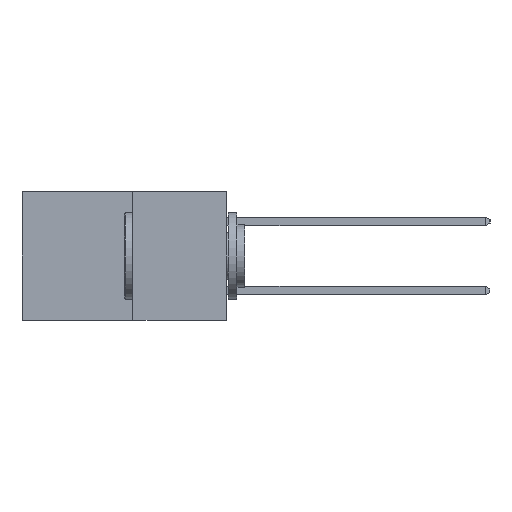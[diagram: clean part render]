
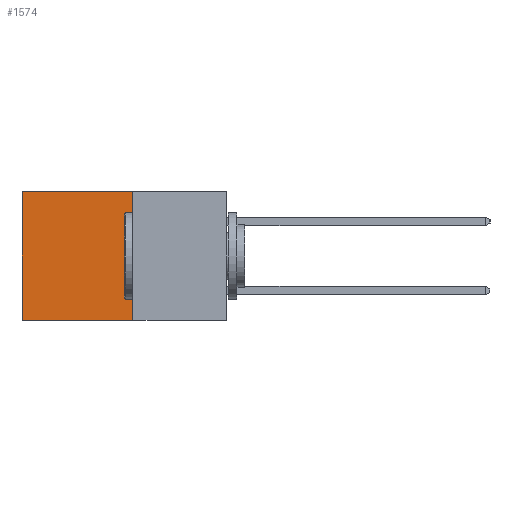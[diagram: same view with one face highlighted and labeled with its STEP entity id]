
A CAD part, left-side view. The second image highlights one B-rep face of the part: STEP entity #1574.
In plain terms, the highlighted planar face has unit normal (-1, 0, 0).
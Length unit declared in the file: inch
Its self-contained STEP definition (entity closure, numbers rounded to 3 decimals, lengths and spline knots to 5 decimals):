
#288 = ORIENTED_EDGE ( 'NONE', *, *, #5386, .F. ) ;
#1240 = VECTOR ( 'NONE', #7402, 39.37008 ) ;
#1245 = EDGE_LOOP ( 'NONE', ( #10589, #288, #12506, #8542 ) ) ;
#1574 = ADVANCED_FACE ( 'NONE', ( #5909 ), #2010, .F. ) ;
#2010 = PLANE ( 'NONE',  #11711 ) ;
#2177 = VECTOR ( 'NONE', #7965, 39.37008 ) ;
#2582 = VERTEX_POINT ( 'NONE', #15142 ) ;
#2954 = VECTOR ( 'NONE', #12446, 39.37008 ) ;
#4867 = LINE ( 'NONE', #7369, #1240 ) ;
#5386 = EDGE_CURVE ( 'NONE', #13841, #8059, #6153, .T. ) ;
#5751 = CARTESIAN_POINT ( 'NONE',  ( 0.277, 0.27, -0.37 ) ) ;
#5849 = EDGE_CURVE ( 'NONE', #2582, #8685, #15281, .T. ) ;
#5909 = FACE_OUTER_BOUND ( 'NONE', #1245, .T. ) ;
#5916 = EDGE_CURVE ( 'NONE', #8685, #8059, #4867, .T. ) ;
#5941 = DIRECTION ( 'NONE',  ( 0., 0., -1. ) ) ;
#6153 = LINE ( 'NONE', #12502, #2954 ) ;
#6568 = CARTESIAN_POINT ( 'NONE',  ( 0.277, 0.59, -0.37 ) ) ;
#6663 = DIRECTION ( 'NONE',  ( 0., 0., -1. ) ) ;
#7369 = CARTESIAN_POINT ( 'NONE',  ( 0.277, 0.59, -0.37 ) ) ;
#7402 = DIRECTION ( 'NONE',  ( 0., 0., -1. ) ) ;
#7678 = CARTESIAN_POINT ( 'NONE',  ( 0.277, 0.27, -0.37 ) ) ;
#7965 = DIRECTION ( 'NONE',  ( 0., 1., 0. ) ) ;
#8037 = CARTESIAN_POINT ( 'NONE',  ( 0.277, 0.27, 0. ) ) ;
#8059 = VERTEX_POINT ( 'NONE', #6568 ) ;
#8542 = ORIENTED_EDGE ( 'NONE', *, *, #5849, .T. ) ;
#8668 = LINE ( 'NONE', #11528, #9056 ) ;
#8685 = VERTEX_POINT ( 'NONE', #9163 ) ;
#9056 = VECTOR ( 'NONE', #6663, 39.37008 ) ;
#9163 = CARTESIAN_POINT ( 'NONE',  ( 0.277, 0.59, 0. ) ) ;
#10589 = ORIENTED_EDGE ( 'NONE', *, *, #5916, .T. ) ;
#11528 = CARTESIAN_POINT ( 'NONE',  ( 0.277, 0.27, -0.37 ) ) ;
#11711 = AXIS2_PLACEMENT_3D ( 'NONE', #7678, #11912, #5941 ) ;
#11912 = DIRECTION ( 'NONE',  ( 1., 0., 0. ) ) ;
#12446 = DIRECTION ( 'NONE',  ( 0., 1., 0. ) ) ;
#12502 = CARTESIAN_POINT ( 'NONE',  ( 0.277, 0.27, -0.37 ) ) ;
#12506 = ORIENTED_EDGE ( 'NONE', *, *, #14345, .F. ) ;
#13841 = VERTEX_POINT ( 'NONE', #5751 ) ;
#14345 = EDGE_CURVE ( 'NONE', #2582, #13841, #8668, .T. ) ;
#15142 = CARTESIAN_POINT ( 'NONE',  ( 0.277, 0.27, 0. ) ) ;
#15281 = LINE ( 'NONE', #8037, #2177 ) ;
